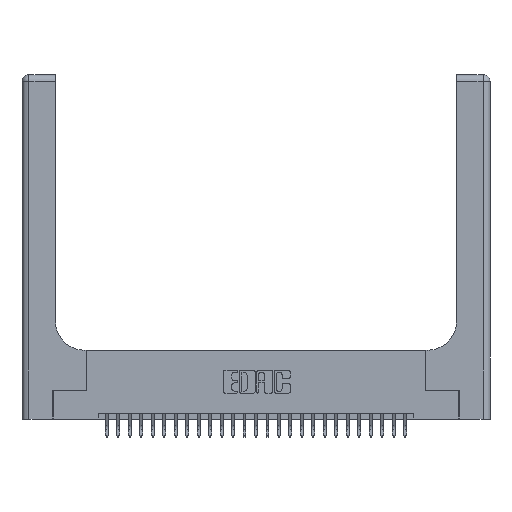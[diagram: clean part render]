
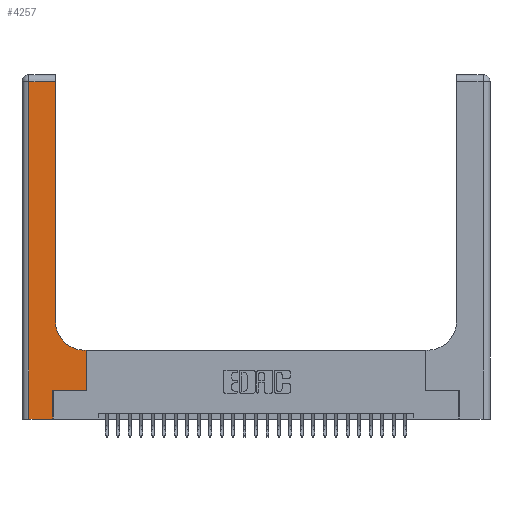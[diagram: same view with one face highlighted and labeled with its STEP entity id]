
A CAD part, top view. The second image highlights one B-rep face of the part: STEP entity #4257.
In plain terms, the highlighted planar face has unit normal (0, 0, 1).
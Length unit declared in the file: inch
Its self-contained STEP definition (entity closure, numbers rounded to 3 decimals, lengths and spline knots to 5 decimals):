
#1268 = CARTESIAN_POINT ( 'NONE',  ( 0.5415, 0.6, 0.37 ) ) ;
#2099 = DIRECTION ( 'NONE',  ( -1., 0., 0. ) ) ;
#2721 = EDGE_CURVE ( 'NONE', #16979, #3666, #9899, .T. ) ;
#2759 = VERTEX_POINT ( 'NONE', #10980 ) ;
#2806 = VECTOR ( 'NONE', #22730, 39.37008 ) ;
#2972 = CARTESIAN_POINT ( 'NONE',  ( 0.269, 0.25, 0.37 ) ) ;
#3068 = VERTEX_POINT ( 'NONE', #3106 ) ;
#3106 = CARTESIAN_POINT ( 'NONE',  ( 0.06, 2.94, 0.37 ) ) ;
#3520 = LINE ( 'NONE', #27071, #2806 ) ;
#3539 = DIRECTION ( 'NONE',  ( 0., 1., 0. ) ) ;
#3666 = VERTEX_POINT ( 'NONE', #7591 ) ;
#3674 = EDGE_CURVE ( 'NONE', #11658, #25444, #8449, .T. ) ;
#3800 = EDGE_CURVE ( 'NONE', #2759, #22348, #11560, .T. ) ;
#4257 = ADVANCED_FACE ( 'NONE', ( #16072 ), #18324, .F. ) ;
#4572 = EDGE_CURVE ( 'NONE', #3068, #23839, #13608, .T. ) ;
#5058 = LINE ( 'NONE', #13232, #10330 ) ;
#5564 = CARTESIAN_POINT ( 'NONE',  ( 0.269, 0., 0.37 ) ) ;
#5568 = ORIENTED_EDGE ( 'NONE', *, *, #4572, .T. ) ;
#6279 = ORIENTED_EDGE ( 'NONE', *, *, #12446, .T. ) ;
#6623 = CARTESIAN_POINT ( 'NONE',  ( 0.269, 0.25, 0.37 ) ) ;
#7268 = CARTESIAN_POINT ( 'NONE',  ( 0., 3., 0.37 ) ) ;
#7591 = CARTESIAN_POINT ( 'NONE',  ( 0.2915, 0.85, 0.37 ) ) ;
#7972 = CARTESIAN_POINT ( 'NONE',  ( 0., 2.94, 0.37 ) ) ;
#8449 = LINE ( 'NONE', #9828, #20868 ) ;
#8633 = DIRECTION ( 'NONE',  ( 0., 0., -1. ) ) ;
#9156 = VECTOR ( 'NONE', #11660, 39.37008 ) ;
#9446 = CARTESIAN_POINT ( 'NONE',  ( 0., 0., 0.37 ) ) ;
#9828 = CARTESIAN_POINT ( 'NONE',  ( 0.269, 0., 0.37 ) ) ;
#9899 = CIRCLE ( 'NONE', #10514, 0.25 ) ;
#10330 = VECTOR ( 'NONE', #2099, 39.37008 ) ;
#10514 = AXIS2_PLACEMENT_3D ( 'NONE', #21829, #8633, #24002 ) ;
#10720 = AXIS2_PLACEMENT_3D ( 'NONE', #7268, #11726, #26999 ) ;
#10980 = CARTESIAN_POINT ( 'NONE',  ( 0.5585, 0.25, 0.37 ) ) ;
#11396 = ORIENTED_EDGE ( 'NONE', *, *, #13274, .T. ) ;
#11560 = LINE ( 'NONE', #14694, #21878 ) ;
#11634 = CARTESIAN_POINT ( 'NONE',  ( 0.5585, 0.6, 0.37 ) ) ;
#11658 = VERTEX_POINT ( 'NONE', #5564 ) ;
#11660 = DIRECTION ( 'NONE',  ( 1., 0., 0. ) ) ;
#11726 = DIRECTION ( 'NONE',  ( 0., 0., -1. ) ) ;
#11987 = CARTESIAN_POINT ( 'NONE',  ( 0.2915, 2.94, 0.37 ) ) ;
#12040 = LINE ( 'NONE', #6623, #17952 ) ;
#12446 = EDGE_CURVE ( 'NONE', #3666, #12496, #3520, .T. ) ;
#12496 = VERTEX_POINT ( 'NONE', #11987 ) ;
#13232 = CARTESIAN_POINT ( 'NONE',  ( 0.2915, 0.6, 0.37 ) ) ;
#13250 = DIRECTION ( 'NONE',  ( 1., 0., 0. ) ) ;
#13274 = EDGE_CURVE ( 'NONE', #12496, #3068, #15349, .T. ) ;
#13514 = ORIENTED_EDGE ( 'NONE', *, *, #20590, .T. ) ;
#13608 = LINE ( 'NONE', #21806, #25889 ) ;
#14694 = CARTESIAN_POINT ( 'NONE',  ( 0.5585, 0.25, 0.37 ) ) ;
#15349 = LINE ( 'NONE', #7972, #20469 ) ;
#15774 = LINE ( 'NONE', #9446, #9156 ) ;
#16072 = FACE_OUTER_BOUND ( 'NONE', #20635, .T. ) ;
#16819 = ORIENTED_EDGE ( 'NONE', *, *, #21444, .T. ) ;
#16979 = VERTEX_POINT ( 'NONE', #1268 ) ;
#17505 = CARTESIAN_POINT ( 'NONE',  ( 0.06, 0., 0.37 ) ) ;
#17952 = VECTOR ( 'NONE', #13250, 39.37008 ) ;
#18324 = PLANE ( 'NONE',  #10720 ) ;
#19566 = ORIENTED_EDGE ( 'NONE', *, *, #3800, .T. ) ;
#19627 = DIRECTION ( 'NONE',  ( 0., -1., 0. ) ) ;
#20469 = VECTOR ( 'NONE', #25529, 39.37008 ) ;
#20590 = EDGE_CURVE ( 'NONE', #22348, #16979, #5058, .T. ) ;
#20635 = EDGE_LOOP ( 'NONE', ( #6279, #11396, #5568, #25863, #26924, #16819, #19566, #13514, #25101 ) ) ;
#20868 = VECTOR ( 'NONE', #27321, 39.37008 ) ;
#21444 = EDGE_CURVE ( 'NONE', #25444, #2759, #12040, .T. ) ;
#21806 = CARTESIAN_POINT ( 'NONE',  ( 0.06, 3., 0.37 ) ) ;
#21829 = CARTESIAN_POINT ( 'NONE',  ( 0.5415, 0.85, 0.37 ) ) ;
#21878 = VECTOR ( 'NONE', #3539, 39.37008 ) ;
#22348 = VERTEX_POINT ( 'NONE', #11634 ) ;
#22730 = DIRECTION ( 'NONE',  ( 0., 1., 0. ) ) ;
#23839 = VERTEX_POINT ( 'NONE', #17505 ) ;
#24002 = DIRECTION ( 'NONE',  ( 1., 0., 0. ) ) ;
#25101 = ORIENTED_EDGE ( 'NONE', *, *, #2721, .T. ) ;
#25444 = VERTEX_POINT ( 'NONE', #2972 ) ;
#25529 = DIRECTION ( 'NONE',  ( -1., 0., 0. ) ) ;
#25863 = ORIENTED_EDGE ( 'NONE', *, *, #27400, .T. ) ;
#25889 = VECTOR ( 'NONE', #19627, 39.37008 ) ;
#26924 = ORIENTED_EDGE ( 'NONE', *, *, #3674, .T. ) ;
#26999 = DIRECTION ( 'NONE',  ( -1., 0., 0. ) ) ;
#27071 = CARTESIAN_POINT ( 'NONE',  ( 0.2915, 3., 0.37 ) ) ;
#27321 = DIRECTION ( 'NONE',  ( 0., 1., 0. ) ) ;
#27400 = EDGE_CURVE ( 'NONE', #23839, #11658, #15774, .T. ) ;
